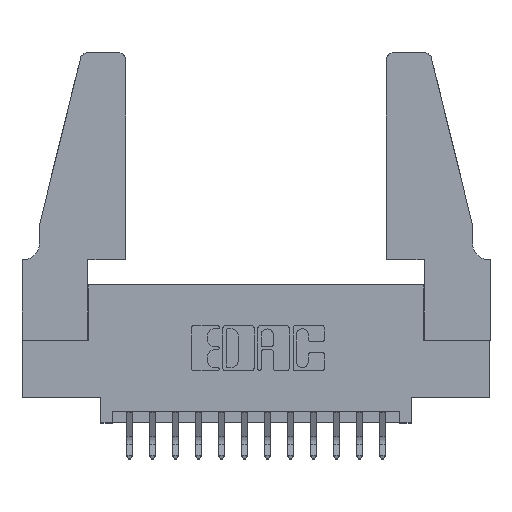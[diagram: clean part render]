
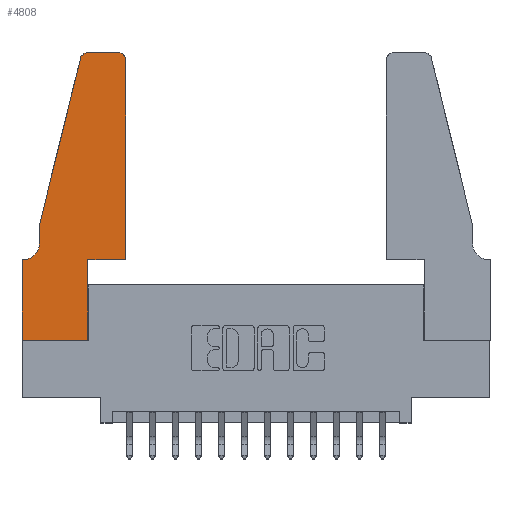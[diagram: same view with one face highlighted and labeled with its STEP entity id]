
A CAD part, top view. The second image highlights one B-rep face of the part: STEP entity #4808.
In plain terms, the highlighted planar face has unit normal (0, 0, 1).
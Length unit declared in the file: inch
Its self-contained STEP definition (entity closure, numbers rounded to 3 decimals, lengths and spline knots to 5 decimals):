
#121 = DIRECTION ( 'NONE',  ( 0., -1., 0. ) ) ;
#127 = AXIS2_PLACEMENT_3D ( 'NONE', #10046, #525, #136 ) ;
#136 = DIRECTION ( 'NONE',  ( 1., 0., 0. ) ) ;
#468 = VECTOR ( 'NONE', #8658, 39.37008 ) ;
#525 = DIRECTION ( 'NONE',  ( 0., 0., 1. ) ) ;
#597 = VECTOR ( 'NONE', #7333, 39.37008 ) ;
#689 = CARTESIAN_POINT ( 'NONE',  ( 0.2605, 1.25, 0.37 ) ) ;
#742 = VECTOR ( 'NONE', #5606, 39.37008 ) ;
#850 = EDGE_CURVE ( 'NONE', #1687, #8391, #9970, .T. ) ;
#878 = CARTESIAN_POINT ( 'NONE',  ( 0., 0., 0.37 ) ) ;
#949 = VECTOR ( 'NONE', #15032, 39.37008 ) ;
#966 = VERTEX_POINT ( 'NONE', #12944 ) ;
#1071 = DIRECTION ( 'NONE',  ( 0., 0., -1. ) ) ;
#1242 = VERTEX_POINT ( 'NONE', #878 ) ;
#1295 = ORIENTED_EDGE ( 'NONE', *, *, #2700, .T. ) ;
#1529 = VECTOR ( 'NONE', #2190, 39.37008 ) ;
#1572 = CARTESIAN_POINT ( 'NONE',  ( 0.4505, 1.22, 0.37 ) ) ;
#1616 = LINE ( 'NONE', #689, #14722 ) ;
#1678 = ORIENTED_EDGE ( 'NONE', *, *, #6246, .T. ) ;
#1687 = VERTEX_POINT ( 'NONE', #1572 ) ;
#1832 = CARTESIAN_POINT ( 'NONE',  ( 0.284, 1.25, 0.37 ) ) ;
#2186 = CARTESIAN_POINT ( 'NONE',  ( 0.284, 1.22, 0.37 ) ) ;
#2190 = DIRECTION ( 'NONE',  ( 1., 0., 0. ) ) ;
#2700 = EDGE_CURVE ( 'NONE', #5406, #1242, #3313, .T. ) ;
#2731 = CIRCLE ( 'NONE', #13178, 0.03 ) ;
#3177 = DIRECTION ( 'NONE',  ( -1., 0., 0. ) ) ;
#3266 = DIRECTION ( 'NONE',  ( -0.239, -0.971, 0. ) ) ;
#3313 = LINE ( 'NONE', #10051, #13529 ) ;
#3462 = DIRECTION ( 'NONE',  ( 1., 0., 0. ) ) ;
#3750 = CARTESIAN_POINT ( 'NONE',  ( 0.2865, 0., 0.37 ) ) ;
#3809 = VERTEX_POINT ( 'NONE', #12057 ) ;
#3825 = VERTEX_POINT ( 'NONE', #12108 ) ;
#4331 = VERTEX_POINT ( 'NONE', #10682 ) ;
#4425 = CARTESIAN_POINT ( 'NONE',  ( 0., 0.35, 0.37 ) ) ;
#4479 = FACE_OUTER_BOUND ( 'NONE', #15626, .T. ) ;
#4808 = ADVANCED_FACE ( 'NONE', ( #4479 ), #5630, .T. ) ;
#5225 = CARTESIAN_POINT ( 'NONE',  ( 0.2865, 0.35, 0.37 ) ) ;
#5406 = VERTEX_POINT ( 'NONE', #4425 ) ;
#5442 = VECTOR ( 'NONE', #6670, 39.37008 ) ;
#5553 = EDGE_CURVE ( 'NONE', #3809, #3825, #12903, .T. ) ;
#5606 = DIRECTION ( 'NONE',  ( 0., -1., 0. ) ) ;
#5630 = PLANE ( 'NONE',  #9160 ) ;
#5758 = AXIS2_PLACEMENT_3D ( 'NONE', #8516, #1071, #9741 ) ;
#5950 = VERTEX_POINT ( 'NONE', #8174 ) ;
#6246 = EDGE_CURVE ( 'NONE', #1242, #13984, #7088, .T. ) ;
#6349 = ORIENTED_EDGE ( 'NONE', *, *, #7310, .T. ) ;
#6670 = DIRECTION ( 'NONE',  ( -1., 0., 0. ) ) ;
#6738 = ORIENTED_EDGE ( 'NONE', *, *, #8141, .T. ) ;
#6892 = CARTESIAN_POINT ( 'NONE',  ( 0.25487, 1.22718, 0.37 ) ) ;
#7088 = LINE ( 'NONE', #11075, #468 ) ;
#7133 = ORIENTED_EDGE ( 'NONE', *, *, #13651, .T. ) ;
#7294 = VERTEX_POINT ( 'NONE', #6892 ) ;
#7310 = EDGE_CURVE ( 'NONE', #8391, #15736, #1616, .T. ) ;
#7333 = DIRECTION ( 'NONE',  ( 0., 1., 0. ) ) ;
#7522 = ORIENTED_EDGE ( 'NONE', *, *, #9755, .T. ) ;
#8095 = CARTESIAN_POINT ( 'NONE',  ( 0.0755, 0.5, 0.37 ) ) ;
#8117 = DIRECTION ( 'NONE',  ( 1., 0., 0. ) ) ;
#8141 = EDGE_CURVE ( 'NONE', #15736, #7294, #2731, .T. ) ;
#8174 = CARTESIAN_POINT ( 'NONE',  ( 0.0755, 0.5, 0.37 ) ) ;
#8391 = VERTEX_POINT ( 'NONE', #10265 ) ;
#8516 = CARTESIAN_POINT ( 'NONE',  ( 0.0055, 0.42, 0.37 ) ) ;
#8658 = DIRECTION ( 'NONE',  ( 1., 0., 0. ) ) ;
#8736 = LINE ( 'NONE', #10334, #5442 ) ;
#9160 = AXIS2_PLACEMENT_3D ( 'NONE', #14187, #15440, #8117 ) ;
#9313 = LINE ( 'NONE', #15539, #12187 ) ;
#9639 = CARTESIAN_POINT ( 'NONE',  ( 0.4505, 0.35, 0.37 ) ) ;
#9741 = DIRECTION ( 'NONE',  ( -1., 0., 0. ) ) ;
#9755 = EDGE_CURVE ( 'NONE', #3825, #5406, #8736, .T. ) ;
#9970 = CIRCLE ( 'NONE', #127, 0.03 ) ;
#10046 = CARTESIAN_POINT ( 'NONE',  ( 0.4205, 1.22, 0.37 ) ) ;
#10050 = EDGE_CURVE ( 'NONE', #4331, #966, #11035, .T. ) ;
#10051 = CARTESIAN_POINT ( 'NONE',  ( 0., 0., 0.37 ) ) ;
#10265 = CARTESIAN_POINT ( 'NONE',  ( 0.4205, 1.25, 0.37 ) ) ;
#10334 = CARTESIAN_POINT ( 'NONE',  ( 0.0755, 0.35, 0.37 ) ) ;
#10404 = ORIENTED_EDGE ( 'NONE', *, *, #5553, .T. ) ;
#10438 = LINE ( 'NONE', #5225, #949 ) ;
#10484 = LINE ( 'NONE', #11090, #597 ) ;
#10682 = CARTESIAN_POINT ( 'NONE',  ( 0.2865, 0.35, 0.37 ) ) ;
#10869 = DIRECTION ( 'NONE',  ( 0., 0., 1. ) ) ;
#11035 = LINE ( 'NONE', #9639, #1529 ) ;
#11075 = CARTESIAN_POINT ( 'NONE',  ( 0., 0., 0.37 ) ) ;
#11090 = CARTESIAN_POINT ( 'NONE',  ( 0.4505, 0.35, 0.37 ) ) ;
#12057 = CARTESIAN_POINT ( 'NONE',  ( 0.0755, 0.42, 0.37 ) ) ;
#12108 = CARTESIAN_POINT ( 'NONE',  ( 0.0055, 0.35, 0.37 ) ) ;
#12116 = EDGE_CURVE ( 'NONE', #966, #1687, #10484, .T. ) ;
#12187 = VECTOR ( 'NONE', #3266, 39.37008 ) ;
#12325 = ORIENTED_EDGE ( 'NONE', *, *, #12116, .T. ) ;
#12903 = CIRCLE ( 'NONE', #5758, 0.07 ) ;
#12944 = CARTESIAN_POINT ( 'NONE',  ( 0.4505, 0.35, 0.37 ) ) ;
#13060 = EDGE_CURVE ( 'NONE', #7294, #5950, #9313, .T. ) ;
#13178 = AXIS2_PLACEMENT_3D ( 'NONE', #2186, #10869, #3462 ) ;
#13266 = ORIENTED_EDGE ( 'NONE', *, *, #13060, .T. ) ;
#13431 = EDGE_CURVE ( 'NONE', #13984, #4331, #10438, .T. ) ;
#13529 = VECTOR ( 'NONE', #121, 39.37008 ) ;
#13651 = EDGE_CURVE ( 'NONE', #5950, #3809, #13854, .T. ) ;
#13854 = LINE ( 'NONE', #8095, #742 ) ;
#13984 = VERTEX_POINT ( 'NONE', #3750 ) ;
#14187 = CARTESIAN_POINT ( 'NONE',  ( 0., 0.35, 0.37 ) ) ;
#14722 = VECTOR ( 'NONE', #3177, 39.37008 ) ;
#14784 = ORIENTED_EDGE ( 'NONE', *, *, #13431, .T. ) ;
#15032 = DIRECTION ( 'NONE',  ( 0., 1., 0. ) ) ;
#15172 = ORIENTED_EDGE ( 'NONE', *, *, #10050, .T. ) ;
#15440 = DIRECTION ( 'NONE',  ( 0., 0., 1. ) ) ;
#15539 = CARTESIAN_POINT ( 'NONE',  ( 0.0755, 0.5, 0.37 ) ) ;
#15566 = ORIENTED_EDGE ( 'NONE', *, *, #850, .T. ) ;
#15626 = EDGE_LOOP ( 'NONE', ( #6349, #6738, #13266, #7133, #10404, #7522, #1295, #1678, #14784, #15172, #12325, #15566 ) ) ;
#15736 = VERTEX_POINT ( 'NONE', #1832 ) ;
